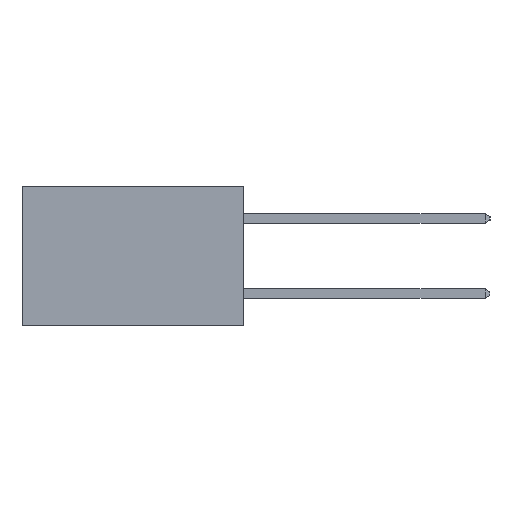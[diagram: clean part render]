
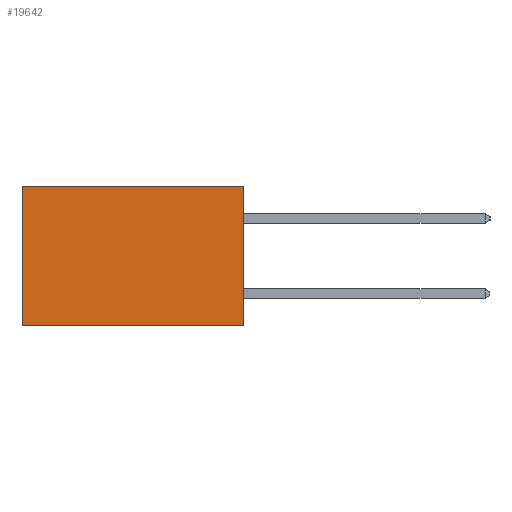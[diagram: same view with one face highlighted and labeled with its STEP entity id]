
A CAD part, left-side view. The second image highlights one B-rep face of the part: STEP entity #19642.
In plain terms, the highlighted planar face has unit normal (-1, 0, 0).
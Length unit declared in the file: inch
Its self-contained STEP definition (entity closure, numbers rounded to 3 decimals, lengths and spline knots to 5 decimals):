
#840 = CARTESIAN_POINT ( 'NONE',  ( 0.277, 0., -0.37 ) ) ;
#1706 = DIRECTION ( 'NONE',  ( 0., 0., -1. ) ) ;
#2120 = CARTESIAN_POINT ( 'NONE',  ( 0.277, 0., -0.37 ) ) ;
#2612 = PLANE ( 'NONE',  #8569 ) ;
#2953 = VECTOR ( 'NONE', #4966, 39.37008 ) ;
#2987 = VERTEX_POINT ( 'NONE', #9124 ) ;
#3376 = VECTOR ( 'NONE', #14732, 39.37008 ) ;
#3904 = LINE ( 'NONE', #8224, #3376 ) ;
#4311 = DIRECTION ( 'NONE',  ( 1., 0., 0. ) ) ;
#4966 = DIRECTION ( 'NONE',  ( 0., 1., 0. ) ) ;
#6483 = VERTEX_POINT ( 'NONE', #17840 ) ;
#7191 = FACE_OUTER_BOUND ( 'NONE', #20148, .T. ) ;
#8224 = CARTESIAN_POINT ( 'NONE',  ( 0.277, 0., -0.37 ) ) ;
#8569 = AXIS2_PLACEMENT_3D ( 'NONE', #840, #4311, #15825 ) ;
#9124 = CARTESIAN_POINT ( 'NONE',  ( 0.277, 0., 0. ) ) ;
#9510 = VECTOR ( 'NONE', #1706, 39.37008 ) ;
#10137 = VERTEX_POINT ( 'NONE', #2120 ) ;
#11404 = DIRECTION ( 'NONE',  ( 0., 0., -1. ) ) ;
#11468 = LINE ( 'NONE', #19576, #15327 ) ;
#11597 = CARTESIAN_POINT ( 'NONE',  ( 0.277, 0.59, -0.37 ) ) ;
#11677 = CARTESIAN_POINT ( 'NONE',  ( 0.277, 0., -0.37 ) ) ;
#13332 = LINE ( 'NONE', #11677, #9510 ) ;
#13429 = VERTEX_POINT ( 'NONE', #11597 ) ;
#13453 = EDGE_CURVE ( 'NONE', #2987, #10137, #13332, .T. ) ;
#14103 = EDGE_CURVE ( 'NONE', #2987, #6483, #18946, .T. ) ;
#14732 = DIRECTION ( 'NONE',  ( 0., 1., 0. ) ) ;
#14754 = EDGE_CURVE ( 'NONE', #6483, #13429, #11468, .T. ) ;
#15327 = VECTOR ( 'NONE', #11404, 39.37008 ) ;
#15825 = DIRECTION ( 'NONE',  ( 0., 0., -1. ) ) ;
#16462 = CARTESIAN_POINT ( 'NONE',  ( 0.277, 0., 0. ) ) ;
#17840 = CARTESIAN_POINT ( 'NONE',  ( 0.277, 0.59, 0. ) ) ;
#17852 = EDGE_CURVE ( 'NONE', #10137, #13429, #3904, .T. ) ;
#18946 = LINE ( 'NONE', #16462, #2953 ) ;
#19576 = CARTESIAN_POINT ( 'NONE',  ( 0.277, 0.59, -0.37 ) ) ;
#19642 = ADVANCED_FACE ( 'NONE', ( #7191 ), #2612, .F. ) ;
#20148 = EDGE_LOOP ( 'NONE', ( #20430, #21176, #21266, #20799 ) ) ;
#20430 = ORIENTED_EDGE ( 'NONE', *, *, #14754, .T. ) ;
#20799 = ORIENTED_EDGE ( 'NONE', *, *, #14103, .T. ) ;
#21176 = ORIENTED_EDGE ( 'NONE', *, *, #17852, .F. ) ;
#21266 = ORIENTED_EDGE ( 'NONE', *, *, #13453, .F. ) ;
